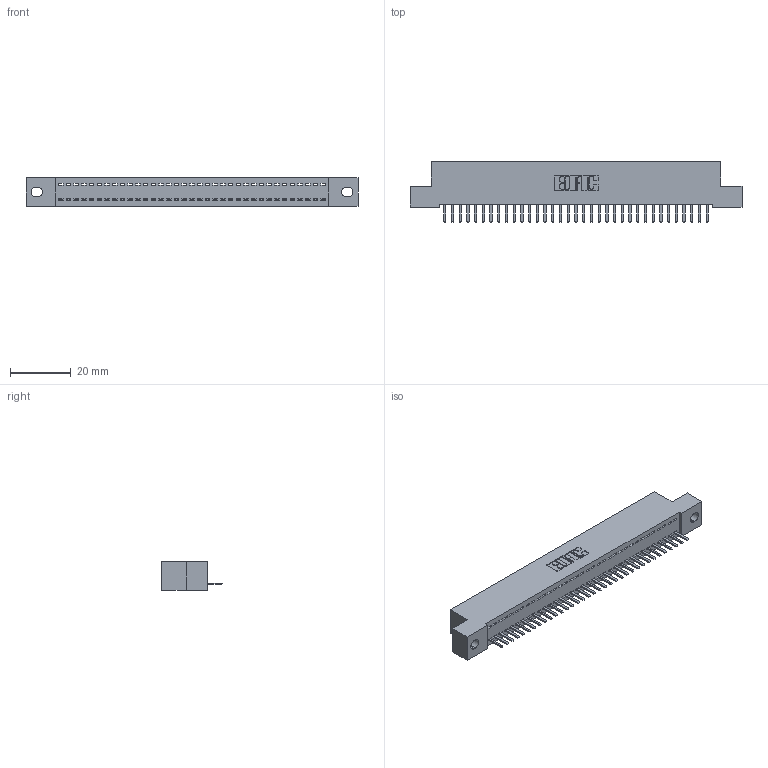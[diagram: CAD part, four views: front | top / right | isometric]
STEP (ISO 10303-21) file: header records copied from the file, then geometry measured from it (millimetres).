
FILE_DESCRIPTION (( 'STEP AP203' ), '1' );
FILE_NAME ('342-035-520-102.STEP', '2018-08-11T19:14:55', ( '' ), ( '' ), 'SwSTEP 2.0', 'SolidWorks 2016', '' );
FILE_SCHEMA (( 'CONFIG_CONTROL_DESIGN' ));
Length unit declared in the file: inch
Products named in the file (3): 345-292-001_345-293-120; 342-035-520-102; 342 Part_.128 Slot
Assembly tree (36 placements, depth 2):
  342-035-520-102
    342 Part_.128 Slot
    345-292-001_345-293-120  x35
Bounding box: 109.22 x 20.02 x 9.4 mm (x, y, z)
Volume: 9397.8 mm3; surface area: 13107.2 mm2
Topology: 36 solids, 36 shells, 2284 faces, 6751 edges, 4406 vertices
Faces by surface type: plane 1610, cylinder 674
Entity records: 22419 total; most frequent: CARTESIAN_POINT 3887, ORIENTED_EDGE 3846, DIRECTION 3281, EDGE_CURVE 1923, LINE 1791, VECTOR 1791, VERTEX_POINT 1278, AXIS2_PLACEMENT_3D 745
